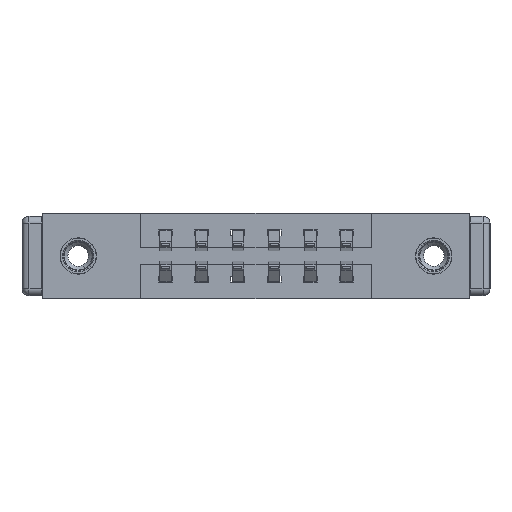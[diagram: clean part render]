
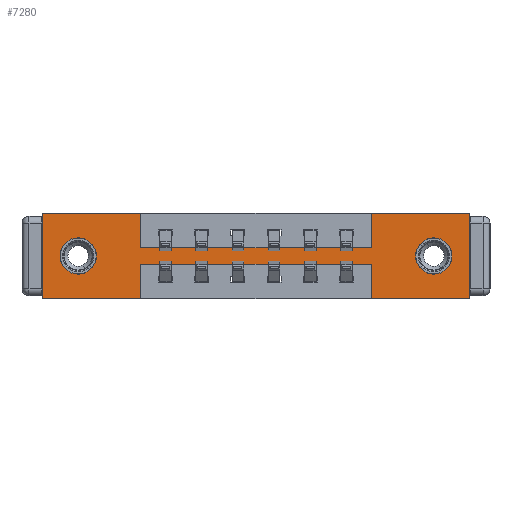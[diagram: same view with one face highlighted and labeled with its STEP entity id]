
A CAD part, front view. The second image highlights one B-rep face of the part: STEP entity #7280.
In plain terms, the highlighted planar face has unit normal (0, -1, 0).
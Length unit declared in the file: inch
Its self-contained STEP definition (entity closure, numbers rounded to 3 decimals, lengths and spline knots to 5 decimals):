
#192 = CARTESIAN_POINT ( 'NONE',  ( 0., 0., -0.37 ) ) ;
#317 = CARTESIAN_POINT ( 'NONE',  ( 0.425, 0., -0.37 ) ) ;
#325 = EDGE_CURVE ( 'NONE', #1877, #5567, #8232, .T. ) ;
#392 = AXIS2_PLACEMENT_3D ( 'NONE', #9344, #11247, #4882 ) ;
#569 = DIRECTION ( 'NONE',  ( 0., 0., 1. ) ) ;
#592 = ORIENTED_EDGE ( 'NONE', *, *, #7878, .F. ) ;
#609 = CARTESIAN_POINT ( 'NONE',  ( 1.842, 0., 0. ) ) ;
#832 = VERTEX_POINT ( 'NONE', #3418 ) ;
#886 = CARTESIAN_POINT ( 'NONE',  ( 1.687, 0., -0.263 ) ) ;
#920 = CARTESIAN_POINT ( 'NONE',  ( 1.687, 0., -0.107 ) ) ;
#999 = VECTOR ( 'NONE', #6967, 39.37008 ) ;
#1203 = EDGE_CURVE ( 'NONE', #3370, #7690, #4401, .T. ) ;
#1328 = VECTOR ( 'NONE', #8619, 39.37008 ) ;
#1489 = VERTEX_POINT ( 'NONE', #7193 ) ;
#1525 = VERTEX_POINT ( 'NONE', #8182 ) ;
#1566 = LINE ( 'NONE', #4995, #10240 ) ;
#1877 = VERTEX_POINT ( 'NONE', #7619 ) ;
#1943 = VECTOR ( 'NONE', #4123, 39.37008 ) ;
#2049 = CARTESIAN_POINT ( 'NONE',  ( 0.155, 0., -0.185 ) ) ;
#2141 = EDGE_CURVE ( 'NONE', #7690, #1525, #9675, .T. ) ;
#2210 = EDGE_CURVE ( 'NONE', #9598, #7824, #5842, .T. ) ;
#2281 = DIRECTION ( 'NONE',  ( -1., 0., 0. ) ) ;
#2322 = CARTESIAN_POINT ( 'NONE',  ( 0.155, 0., -0.107 ) ) ;
#2338 = CIRCLE ( 'NONE', #2502, 0.078 ) ;
#2434 = CARTESIAN_POINT ( 'NONE',  ( 1.417, 0., 0. ) ) ;
#2500 = EDGE_LOOP ( 'NONE', ( #7703, #8773, #4192, #8717, #11471, #2551, #7576, #11897, #5891, #592, #5796, #2698 ) ) ;
#2502 = AXIS2_PLACEMENT_3D ( 'NONE', #8158, #2537, #8198 ) ;
#2537 = DIRECTION ( 'NONE',  ( 0., 1., 0. ) ) ;
#2551 = ORIENTED_EDGE ( 'NONE', *, *, #1203, .F. ) ;
#2698 = ORIENTED_EDGE ( 'NONE', *, *, #325, .F. ) ;
#2716 = DIRECTION ( 'NONE',  ( 0., 0., -1. ) ) ;
#2876 = VECTOR ( 'NONE', #6217, 39.37008 ) ;
#3092 = PLANE ( 'NONE',  #5966 ) ;
#3184 = EDGE_CURVE ( 'NONE', #11524, #5718, #2338, .T. ) ;
#3370 = VERTEX_POINT ( 'NONE', #7750 ) ;
#3418 = CARTESIAN_POINT ( 'NONE',  ( 1.417, 0., -0.15 ) ) ;
#3547 = EDGE_CURVE ( 'NONE', #5718, #11524, #7311, .T. ) ;
#3703 = CARTESIAN_POINT ( 'NONE',  ( 0.425, 0., 0. ) ) ;
#3743 = VERTEX_POINT ( 'NONE', #2322 ) ;
#3872 = EDGE_LOOP ( 'NONE', ( #6121, #5302 ) ) ;
#3957 = VERTEX_POINT ( 'NONE', #3703 ) ;
#4123 = DIRECTION ( 'NONE',  ( -1., 0., 0. ) ) ;
#4129 = EDGE_CURVE ( 'NONE', #11651, #1877, #8904, .T. ) ;
#4192 = ORIENTED_EDGE ( 'NONE', *, *, #2210, .F. ) ;
#4211 = CARTESIAN_POINT ( 'NONE',  ( 1.687, 0., -0.185 ) ) ;
#4228 = AXIS2_PLACEMENT_3D ( 'NONE', #4211, #7867, #10785 ) ;
#4339 = LINE ( 'NONE', #8422, #7589 ) ;
#4401 = LINE ( 'NONE', #11413, #1328 ) ;
#4404 = CARTESIAN_POINT ( 'NONE',  ( 0.425, 0., -0.22 ) ) ;
#4614 = EDGE_CURVE ( 'NONE', #1525, #9598, #4339, .T. ) ;
#4719 = EDGE_CURVE ( 'NONE', #10843, #3743, #10536, .T. ) ;
#4811 = VECTOR ( 'NONE', #7888, 39.37008 ) ;
#4882 = DIRECTION ( 'NONE',  ( 0., 0., 1. ) ) ;
#4903 = DIRECTION ( 'NONE',  ( 0., 1., 0. ) ) ;
#4985 = EDGE_CURVE ( 'NONE', #832, #3370, #11541, .T. ) ;
#4995 = CARTESIAN_POINT ( 'NONE',  ( 0.425, 0., -0.22 ) ) ;
#5088 = CIRCLE ( 'NONE', #392, 0.078 ) ;
#5302 = ORIENTED_EDGE ( 'NONE', *, *, #3547, .T. ) ;
#5502 = FACE_OUTER_BOUND ( 'NONE', #2500, .T. ) ;
#5565 = CARTESIAN_POINT ( 'NONE',  ( 1.842, 0., 0. ) ) ;
#5567 = VERTEX_POINT ( 'NONE', #11013 ) ;
#5669 = LINE ( 'NONE', #9662, #999 ) ;
#5718 = VERTEX_POINT ( 'NONE', #886 ) ;
#5796 = ORIENTED_EDGE ( 'NONE', *, *, #6836, .F. ) ;
#5842 = LINE ( 'NONE', #9305, #6401 ) ;
#5881 = DIRECTION ( 'NONE',  ( 0., 0., -1. ) ) ;
#5891 = ORIENTED_EDGE ( 'NONE', *, *, #7640, .F. ) ;
#5950 = LINE ( 'NONE', #9521, #11992 ) ;
#5966 = AXIS2_PLACEMENT_3D ( 'NONE', #192, #7748, #5881 ) ;
#6109 = VECTOR ( 'NONE', #2716, 39.37008 ) ;
#6121 = ORIENTED_EDGE ( 'NONE', *, *, #3184, .T. ) ;
#6217 = DIRECTION ( 'NONE',  ( 1., 0., 0. ) ) ;
#6260 = CARTESIAN_POINT ( 'NONE',  ( 0., 0., 0. ) ) ;
#6308 = CARTESIAN_POINT ( 'NONE',  ( 1.417, 0., -0.22 ) ) ;
#6401 = VECTOR ( 'NONE', #11208, 39.37008 ) ;
#6457 = EDGE_CURVE ( 'NONE', #1489, #832, #5669, .T. ) ;
#6771 = EDGE_CURVE ( 'NONE', #3743, #10843, #5088, .T. ) ;
#6836 = EDGE_CURVE ( 'NONE', #5567, #11179, #5950, .T. ) ;
#6967 = DIRECTION ( 'NONE',  ( 1., 0., 0. ) ) ;
#7112 = VECTOR ( 'NONE', #8123, 39.37008 ) ;
#7193 = CARTESIAN_POINT ( 'NONE',  ( 0.425, 0., -0.15 ) ) ;
#7273 = FACE_BOUND ( 'NONE', #3872, .T. ) ;
#7280 = ADVANCED_FACE ( 'NONE', ( #7273, #8012, #5502 ), #3092, .T. ) ;
#7311 = CIRCLE ( 'NONE', #4228, 0.078 ) ;
#7576 = ORIENTED_EDGE ( 'NONE', *, *, #4985, .F. ) ;
#7589 = VECTOR ( 'NONE', #10260, 39.37008 ) ;
#7619 = CARTESIAN_POINT ( 'NONE',  ( 0.425, 0., -0.37 ) ) ;
#7640 = EDGE_CURVE ( 'NONE', #3957, #1489, #9010, .T. ) ;
#7690 = VERTEX_POINT ( 'NONE', #609 ) ;
#7703 = ORIENTED_EDGE ( 'NONE', *, *, #4129, .F. ) ;
#7748 = DIRECTION ( 'NONE',  ( 0., -1., 0. ) ) ;
#7750 = CARTESIAN_POINT ( 'NONE',  ( 1.417, 0., 0. ) ) ;
#7799 = CARTESIAN_POINT ( 'NONE',  ( 1.417, 0., -0.37 ) ) ;
#7824 = VERTEX_POINT ( 'NONE', #6308 ) ;
#7867 = DIRECTION ( 'NONE',  ( 0., 1., 0. ) ) ;
#7878 = EDGE_CURVE ( 'NONE', #11179, #3957, #11679, .T. ) ;
#7888 = DIRECTION ( 'NONE',  ( 0., 0., -1. ) ) ;
#7985 = ORIENTED_EDGE ( 'NONE', *, *, #6771, .T. ) ;
#8012 = FACE_BOUND ( 'NONE', #11387, .T. ) ;
#8123 = DIRECTION ( 'NONE',  ( 0., 0., -1. ) ) ;
#8158 = CARTESIAN_POINT ( 'NONE',  ( 1.687, 0., -0.185 ) ) ;
#8182 = CARTESIAN_POINT ( 'NONE',  ( 1.842, 0., -0.37 ) ) ;
#8198 = DIRECTION ( 'NONE',  ( 0., 0., -1. ) ) ;
#8232 = LINE ( 'NONE', #10584, #1943 ) ;
#8422 = CARTESIAN_POINT ( 'NONE',  ( 0., 0., -0.37 ) ) ;
#8589 = DIRECTION ( 'NONE',  ( 0., 0., 1. ) ) ;
#8610 = CARTESIAN_POINT ( 'NONE',  ( 0.155, 0., -0.263 ) ) ;
#8619 = DIRECTION ( 'NONE',  ( 1., 0., 0. ) ) ;
#8717 = ORIENTED_EDGE ( 'NONE', *, *, #4614, .F. ) ;
#8773 = ORIENTED_EDGE ( 'NONE', *, *, #10963, .F. ) ;
#8904 = LINE ( 'NONE', #317, #4811 ) ;
#9010 = LINE ( 'NONE', #9016, #7112 ) ;
#9012 = VECTOR ( 'NONE', #569, 39.37008 ) ;
#9016 = CARTESIAN_POINT ( 'NONE',  ( 0.425, 0., 0. ) ) ;
#9090 = ORIENTED_EDGE ( 'NONE', *, *, #4719, .T. ) ;
#9305 = CARTESIAN_POINT ( 'NONE',  ( 1.417, 0., -0.37 ) ) ;
#9344 = CARTESIAN_POINT ( 'NONE',  ( 0.155, 0., -0.185 ) ) ;
#9458 = CARTESIAN_POINT ( 'NONE',  ( 0., 0., 0. ) ) ;
#9521 = CARTESIAN_POINT ( 'NONE',  ( 0., 0., 0. ) ) ;
#9598 = VERTEX_POINT ( 'NONE', #7799 ) ;
#9662 = CARTESIAN_POINT ( 'NONE',  ( 0.425, 0., -0.15 ) ) ;
#9675 = LINE ( 'NONE', #5565, #6109 ) ;
#10240 = VECTOR ( 'NONE', #2281, 39.37008 ) ;
#10260 = DIRECTION ( 'NONE',  ( -1., 0., 0. ) ) ;
#10474 = DIRECTION ( 'NONE',  ( 0., 0., 1. ) ) ;
#10536 = CIRCLE ( 'NONE', #11067, 0.078 ) ;
#10584 = CARTESIAN_POINT ( 'NONE',  ( 0., 0., -0.37 ) ) ;
#10785 = DIRECTION ( 'NONE',  ( 0., 0., -1. ) ) ;
#10843 = VERTEX_POINT ( 'NONE', #8610 ) ;
#10963 = EDGE_CURVE ( 'NONE', #7824, #11651, #1566, .T. ) ;
#11013 = CARTESIAN_POINT ( 'NONE',  ( 0., 0., -0.37 ) ) ;
#11067 = AXIS2_PLACEMENT_3D ( 'NONE', #2049, #4903, #8589 ) ;
#11179 = VERTEX_POINT ( 'NONE', #9458 ) ;
#11208 = DIRECTION ( 'NONE',  ( 0., 0., 1. ) ) ;
#11247 = DIRECTION ( 'NONE',  ( 0., 1., 0. ) ) ;
#11387 = EDGE_LOOP ( 'NONE', ( #7985, #9090 ) ) ;
#11413 = CARTESIAN_POINT ( 'NONE',  ( 0., 0., 0. ) ) ;
#11471 = ORIENTED_EDGE ( 'NONE', *, *, #2141, .F. ) ;
#11524 = VERTEX_POINT ( 'NONE', #920 ) ;
#11541 = LINE ( 'NONE', #2434, #9012 ) ;
#11651 = VERTEX_POINT ( 'NONE', #4404 ) ;
#11679 = LINE ( 'NONE', #6260, #2876 ) ;
#11897 = ORIENTED_EDGE ( 'NONE', *, *, #6457, .F. ) ;
#11992 = VECTOR ( 'NONE', #10474, 39.37008 ) ;
